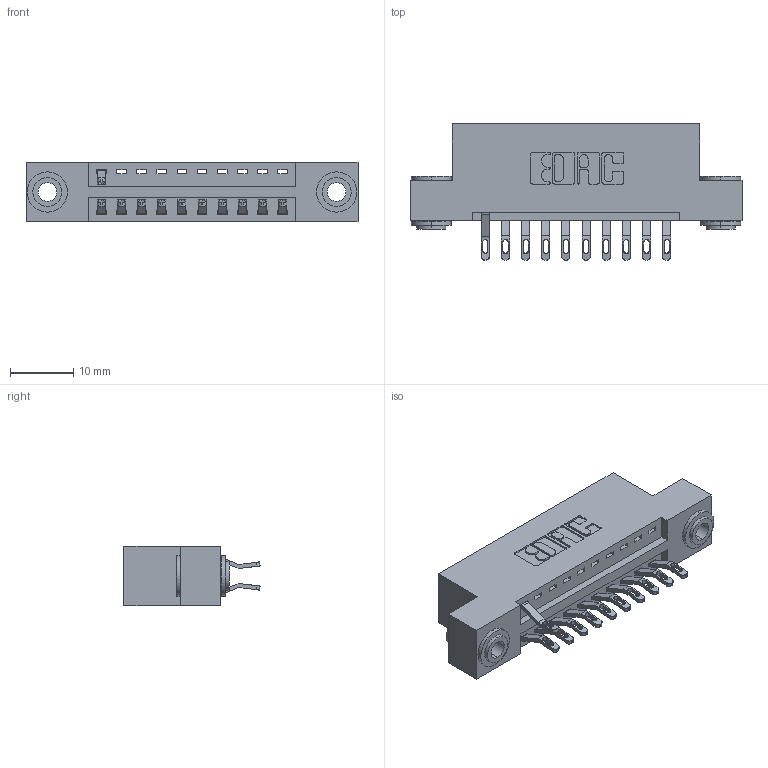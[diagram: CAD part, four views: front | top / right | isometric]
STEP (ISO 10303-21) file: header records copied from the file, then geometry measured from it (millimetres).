
FILE_DESCRIPTION (( 'STEP AP203' ), '1' );
FILE_NAME ('346-020-555-203.STEP', '2018-08-20T21:55:49', ( '' ), ( '' ), 'SwSTEP 2.0', 'SolidWorks 2016', '' );
FILE_SCHEMA (( 'CONFIG_CONTROL_DESIGN' ));
Length unit declared in the file: inch
Products named in the file (4): 346 Part_Flush Mounting Lugs - 0.156 Dia-TH; 345-292-001_555 Tail; 345-250-002_345-250-002-102; 346-020-555-203
Assembly tree (14 placements, depth 2):
  346-020-555-203
    346 Part_Flush Mounting Lugs - 0.156 Dia-TH
    345-292-001_555 Tail  x11
    345-250-002_345-250-002-102  x2
Bounding box: 52.32 x 21.46 x 9.4 mm (x, y, z)
Volume: 4824 mm3; surface area: 5988.8 mm2
Topology: 14 solids, 14 shells, 852 faces, 2607 edges, 1734 vertices
Faces by surface type: plane 494, cylinder 350, cone 8
Entity records: 11522 total; most frequent: CARTESIAN_POINT 1992, ORIENTED_EDGE 1898, DIRECTION 1797, EDGE_CURVE 949, LINE 733, VECTOR 733, VERTEX_POINT 630, AXIS2_PLACEMENT_3D 532
